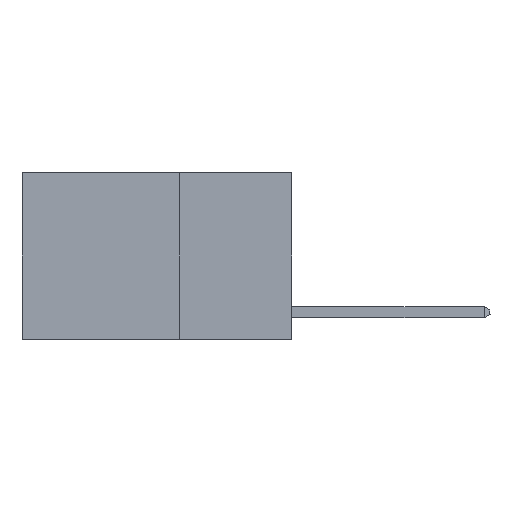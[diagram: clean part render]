
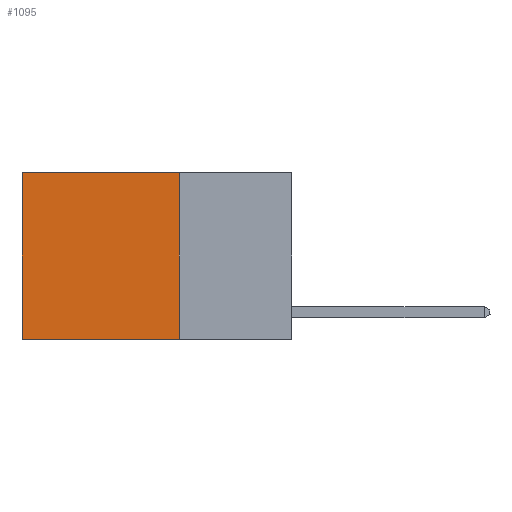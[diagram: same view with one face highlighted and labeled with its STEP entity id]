
A CAD part, left-side view. The second image highlights one B-rep face of the part: STEP entity #1095.
In plain terms, the highlighted planar face has unit normal (-1, 0, 0).
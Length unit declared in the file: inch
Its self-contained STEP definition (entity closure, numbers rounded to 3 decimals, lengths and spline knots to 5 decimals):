
#1046 = EDGE_CURVE ( 'NONE', #5301, #10876, #7341, .T. ) ;
#1095 = ADVANCED_FACE ( 'NONE', ( #3443 ), #10325, .F. ) ;
#1189 = LINE ( 'NONE', #7175, #7981 ) ;
#1319 = DIRECTION ( 'NONE',  ( 0., 1., 0. ) ) ;
#1414 = DIRECTION ( 'NONE',  ( 1., 0., 0. ) ) ;
#1474 = CARTESIAN_POINT ( 'NONE',  ( 0.2625, 0.6, 0. ) ) ;
#1753 = ORIENTED_EDGE ( 'NONE', *, *, #3820, .F. ) ;
#1828 = ORIENTED_EDGE ( 'NONE', *, *, #2844, .F. ) ;
#2844 = EDGE_CURVE ( 'NONE', #7337, #10876, #1189, .T. ) ;
#3408 = CARTESIAN_POINT ( 'NONE',  ( 0.2625, 0.25, 0. ) ) ;
#3443 = FACE_OUTER_BOUND ( 'NONE', #12613, .T. ) ;
#3820 = EDGE_CURVE ( 'NONE', #10105, #7337, #6280, .T. ) ;
#4206 = CARTESIAN_POINT ( 'NONE',  ( 0.2625, 0.25, 0. ) ) ;
#4432 = VECTOR ( 'NONE', #4788, 39.37008 ) ;
#4788 = DIRECTION ( 'NONE',  ( 0., 1., 0. ) ) ;
#5301 = VERTEX_POINT ( 'NONE', #10175 ) ;
#5948 = EDGE_CURVE ( 'NONE', #10105, #5301, #11983, .T. ) ;
#6280 = LINE ( 'NONE', #4206, #10251 ) ;
#7175 = CARTESIAN_POINT ( 'NONE',  ( 0.2625, 0.25, -0.37 ) ) ;
#7337 = VERTEX_POINT ( 'NONE', #10781 ) ;
#7341 = LINE ( 'NONE', #1474, #12477 ) ;
#7591 = CARTESIAN_POINT ( 'NONE',  ( 0.2625, 0.6, -0.37 ) ) ;
#7981 = VECTOR ( 'NONE', #1319, 39.37008 ) ;
#9560 = ORIENTED_EDGE ( 'NONE', *, *, #1046, .T. ) ;
#10105 = VERTEX_POINT ( 'NONE', #3408 ) ;
#10175 = CARTESIAN_POINT ( 'NONE',  ( 0.2625, 0.6, 0. ) ) ;
#10251 = VECTOR ( 'NONE', #11094, 39.37008 ) ;
#10303 = ORIENTED_EDGE ( 'NONE', *, *, #5948, .T. ) ;
#10325 = PLANE ( 'NONE',  #10572 ) ;
#10572 = AXIS2_PLACEMENT_3D ( 'NONE', #12493, #1414, #11367 ) ;
#10781 = CARTESIAN_POINT ( 'NONE',  ( 0.2625, 0.25, -0.37 ) ) ;
#10876 = VERTEX_POINT ( 'NONE', #7591 ) ;
#11094 = DIRECTION ( 'NONE',  ( 0., 0., -1. ) ) ;
#11367 = DIRECTION ( 'NONE',  ( 0., 0., -1. ) ) ;
#11983 = LINE ( 'NONE', #12729, #4432 ) ;
#12477 = VECTOR ( 'NONE', #12568, 39.37008 ) ;
#12493 = CARTESIAN_POINT ( 'NONE',  ( 0.2625, 0.25, 0. ) ) ;
#12568 = DIRECTION ( 'NONE',  ( 0., 0., -1. ) ) ;
#12613 = EDGE_LOOP ( 'NONE', ( #9560, #1828, #1753, #10303 ) ) ;
#12729 = CARTESIAN_POINT ( 'NONE',  ( 0.2625, 0.25, 0. ) ) ;
